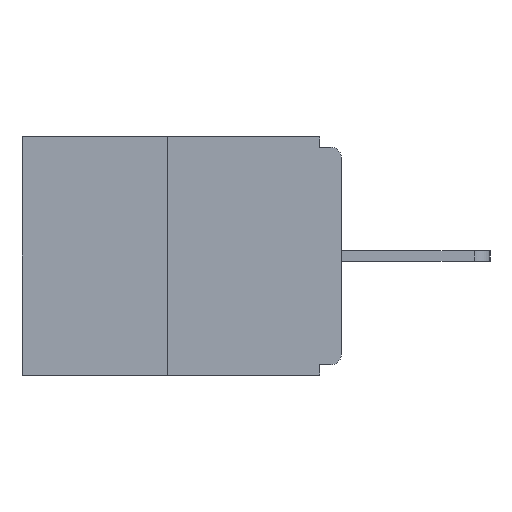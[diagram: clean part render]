
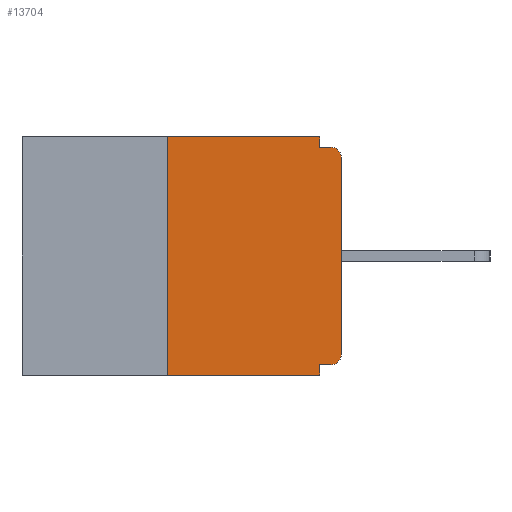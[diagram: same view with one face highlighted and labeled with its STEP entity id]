
A CAD part, left-side view. The second image highlights one B-rep face of the part: STEP entity #13704.
In plain terms, the highlighted planar face has unit normal (-1, 0, 0).
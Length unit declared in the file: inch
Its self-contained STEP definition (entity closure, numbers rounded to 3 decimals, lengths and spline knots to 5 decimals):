
#6 = CARTESIAN_POINT ( 'NONE',  ( 0., 0.25, 0. ) ) ;
#802 = DIRECTION ( 'NONE',  ( 1., 0., 0. ) ) ;
#887 = LINE ( 'NONE', #9673, #11733 ) ;
#1010 = DIRECTION ( 'NONE',  ( 0., -1., 0. ) ) ;
#1548 = EDGE_LOOP ( 'NONE', ( #2287, #24849, #7216, #24230, #19852, #13090, #19005, #3875, #7174, #8209 ) ) ;
#1584 = VERTEX_POINT ( 'NONE', #21967 ) ;
#1664 = EDGE_CURVE ( 'NONE', #17763, #4942, #22661, .T. ) ;
#1900 = VERTEX_POINT ( 'NONE', #4947 ) ;
#1909 = CARTESIAN_POINT ( 'NONE',  ( 0., 0.031, 0. ) ) ;
#2009 = CARTESIAN_POINT ( 'NONE',  ( 0., 0., -0.328 ) ) ;
#2287 = ORIENTED_EDGE ( 'NONE', *, *, #12132, .F. ) ;
#2562 = DIRECTION ( 'NONE',  ( 0., 0., 1. ) ) ;
#2717 = VECTOR ( 'NONE', #25297, 39.37008 ) ;
#2837 = DIRECTION ( 'NONE',  ( -1., 0., 0. ) ) ;
#3025 = DIRECTION ( 'NONE',  ( 0., 0., -1. ) ) ;
#3083 = VERTEX_POINT ( 'NONE', #5964 ) ;
#3099 = LINE ( 'NONE', #24117, #7660 ) ;
#3416 = VECTOR ( 'NONE', #3727, 39.37008 ) ;
#3727 = DIRECTION ( 'NONE',  ( 0., -1., 0. ) ) ;
#3875 = ORIENTED_EDGE ( 'NONE', *, *, #26559, .T. ) ;
#4851 = FACE_OUTER_BOUND ( 'NONE', #1548, .T. ) ;
#4942 = VERTEX_POINT ( 'NONE', #14400 ) ;
#4947 = CARTESIAN_POINT ( 'NONE',  ( 0., 0.015, -0.328 ) ) ;
#5964 = CARTESIAN_POINT ( 'NONE',  ( 0., 0.031, -0.328 ) ) ;
#6010 = VECTOR ( 'NONE', #20680, 39.37008 ) ;
#6138 = VERTEX_POINT ( 'NONE', #14297 ) ;
#6848 = CARTESIAN_POINT ( 'NONE',  ( 0., 0., -0.313 ) ) ;
#7174 = ORIENTED_EDGE ( 'NONE', *, *, #23525, .F. ) ;
#7216 = ORIENTED_EDGE ( 'NONE', *, *, #1664, .T. ) ;
#7660 = VECTOR ( 'NONE', #1010, 39.37008 ) ;
#7672 = EDGE_CURVE ( 'NONE', #1900, #3083, #18581, .T. ) ;
#7760 = CARTESIAN_POINT ( 'NONE',  ( 0., 0.46, -0.343 ) ) ;
#7974 = EDGE_CURVE ( 'NONE', #3083, #4942, #24536, .T. ) ;
#8209 = ORIENTED_EDGE ( 'NONE', *, *, #9772, .F. ) ;
#9386 = DIRECTION ( 'NONE',  ( 0., -1., 0. ) ) ;
#9673 = CARTESIAN_POINT ( 'NONE',  ( 0., 0.46, 0. ) ) ;
#9772 = EDGE_CURVE ( 'NONE', #23815, #15841, #25027, .T. ) ;
#9993 = CARTESIAN_POINT ( 'NONE',  ( 0., 0.031, -0.015 ) ) ;
#10974 = EDGE_CURVE ( 'NONE', #1900, #16771, #22363, .T. ) ;
#11025 = DIRECTION ( 'NONE',  ( 0., 0., -1. ) ) ;
#11733 = VECTOR ( 'NONE', #9386, 39.37008 ) ;
#12132 = EDGE_CURVE ( 'NONE', #17054, #23815, #887, .T. ) ;
#12675 = AXIS2_PLACEMENT_3D ( 'NONE', #20145, #802, #3025 ) ;
#12852 = CARTESIAN_POINT ( 'NONE',  ( 0., 0.031, 0. ) ) ;
#13090 = ORIENTED_EDGE ( 'NONE', *, *, #10974, .T. ) ;
#13257 = DIRECTION ( 'NONE',  ( -1., 0., 0. ) ) ;
#13704 = ADVANCED_FACE ( 'NONE', ( #4851 ), #24330, .F. ) ;
#14221 = VECTOR ( 'NONE', #26599, 39.37008 ) ;
#14297 = CARTESIAN_POINT ( 'NONE',  ( 0., 0.015, -0.015 ) ) ;
#14400 = CARTESIAN_POINT ( 'NONE',  ( 0., 0.031, -0.343 ) ) ;
#14827 = LINE ( 'NONE', #21639, #18078 ) ;
#15079 = CARTESIAN_POINT ( 'NONE',  ( 0., 0.015, -0.03 ) ) ;
#15841 = VERTEX_POINT ( 'NONE', #9993 ) ;
#16771 = VERTEX_POINT ( 'NONE', #6848 ) ;
#17054 = VERTEX_POINT ( 'NONE', #6 ) ;
#17461 = AXIS2_PLACEMENT_3D ( 'NONE', #21907, #2837, #24131 ) ;
#17489 = EDGE_CURVE ( 'NONE', #16771, #1584, #18929, .T. ) ;
#17763 = VERTEX_POINT ( 'NONE', #20147 ) ;
#18078 = VECTOR ( 'NONE', #2562, 39.37008 ) ;
#18581 = LINE ( 'NONE', #2009, #6010 ) ;
#18929 = LINE ( 'NONE', #27397, #20647 ) ;
#19005 = ORIENTED_EDGE ( 'NONE', *, *, #17489, .T. ) ;
#19512 = EDGE_CURVE ( 'NONE', #17763, #17054, #14827, .T. ) ;
#19852 = ORIENTED_EDGE ( 'NONE', *, *, #7672, .F. ) ;
#20145 = CARTESIAN_POINT ( 'NONE',  ( 0., 0.46, 0. ) ) ;
#20147 = CARTESIAN_POINT ( 'NONE',  ( 0., 0.25, -0.343 ) ) ;
#20647 = VECTOR ( 'NONE', #23394, 39.37008 ) ;
#20680 = DIRECTION ( 'NONE',  ( 0., 1., 0. ) ) ;
#21068 = AXIS2_PLACEMENT_3D ( 'NONE', #15079, #13257, #11025 ) ;
#21639 = CARTESIAN_POINT ( 'NONE',  ( 0., 0.25, 0. ) ) ;
#21889 = CARTESIAN_POINT ( 'NONE',  ( 0., 0.031, -0.343 ) ) ;
#21907 = CARTESIAN_POINT ( 'NONE',  ( 0., 0.015, -0.313 ) ) ;
#21967 = CARTESIAN_POINT ( 'NONE',  ( 0., 0., -0.03 ) ) ;
#22363 = CIRCLE ( 'NONE', #17461, 0.015 ) ;
#22661 = LINE ( 'NONE', #7760, #3416 ) ;
#23394 = DIRECTION ( 'NONE',  ( 0., 0., 1. ) ) ;
#23525 = EDGE_CURVE ( 'NONE', #15841, #6138, #3099, .T. ) ;
#23815 = VERTEX_POINT ( 'NONE', #12852 ) ;
#24117 = CARTESIAN_POINT ( 'NONE',  ( 0., 0., -0.015 ) ) ;
#24131 = DIRECTION ( 'NONE',  ( 0., 0., -1. ) ) ;
#24230 = ORIENTED_EDGE ( 'NONE', *, *, #7974, .F. ) ;
#24330 = PLANE ( 'NONE',  #12675 ) ;
#24536 = LINE ( 'NONE', #21889, #14221 ) ;
#24849 = ORIENTED_EDGE ( 'NONE', *, *, #19512, .F. ) ;
#25027 = LINE ( 'NONE', #1909, #2717 ) ;
#25297 = DIRECTION ( 'NONE',  ( 0., 0., -1. ) ) ;
#25953 = CIRCLE ( 'NONE', #21068, 0.015 ) ;
#26559 = EDGE_CURVE ( 'NONE', #1584, #6138, #25953, .T. ) ;
#26599 = DIRECTION ( 'NONE',  ( 0., 0., -1. ) ) ;
#27397 = CARTESIAN_POINT ( 'NONE',  ( 0., 0., 0. ) ) ;
